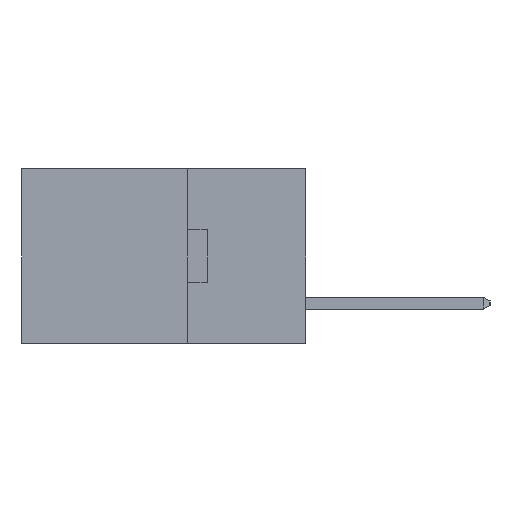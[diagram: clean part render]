
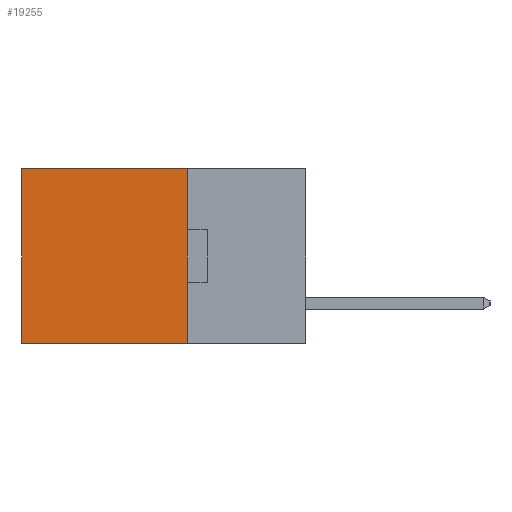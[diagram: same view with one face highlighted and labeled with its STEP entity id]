
A CAD part, left-side view. The second image highlights one B-rep face of the part: STEP entity #19255.
In plain terms, the highlighted planar face has unit normal (-1, 0, 0).
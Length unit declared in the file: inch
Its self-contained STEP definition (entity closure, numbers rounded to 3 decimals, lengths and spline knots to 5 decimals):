
#3061 = VERTEX_POINT ( 'NONE', #18362 ) ;
#4437 = FACE_OUTER_BOUND ( 'NONE', #25617, .T. ) ;
#4675 = CARTESIAN_POINT ( 'NONE',  ( 0.2615, 0.25, -0.37 ) ) ;
#6828 = VERTEX_POINT ( 'NONE', #25820 ) ;
#7215 = EDGE_CURVE ( 'NONE', #6828, #13916, #17630, .T. ) ;
#7653 = EDGE_CURVE ( 'NONE', #15940, #13916, #16345, .T. ) ;
#8813 = PLANE ( 'NONE',  #10673 ) ;
#8828 = ORIENTED_EDGE ( 'NONE', *, *, #11333, .F. ) ;
#10325 = VECTOR ( 'NONE', #12935, 39.37008 ) ;
#10673 = AXIS2_PLACEMENT_3D ( 'NONE', #23127, #10927, #25116 ) ;
#10927 = DIRECTION ( 'NONE',  ( 1., 0., 0. ) ) ;
#11333 = EDGE_CURVE ( 'NONE', #3061, #15940, #19306, .T. ) ;
#11552 = VECTOR ( 'NONE', #21786, 39.37008 ) ;
#12205 = LINE ( 'NONE', #13214, #17010 ) ;
#12935 = DIRECTION ( 'NONE',  ( 0., 0., -1. ) ) ;
#13214 = CARTESIAN_POINT ( 'NONE',  ( 0.2615, 0.25, 0. ) ) ;
#13916 = VERTEX_POINT ( 'NONE', #17057 ) ;
#15294 = DIRECTION ( 'NONE',  ( 0., 1., 0. ) ) ;
#15366 = ORIENTED_EDGE ( 'NONE', *, *, #24944, .T. ) ;
#15718 = VECTOR ( 'NONE', #16014, 39.37008 ) ;
#15844 = CARTESIAN_POINT ( 'NONE',  ( 0.2615, 0.25, -0.37 ) ) ;
#15940 = VERTEX_POINT ( 'NONE', #16402 ) ;
#16014 = DIRECTION ( 'NONE',  ( 0., 1., 0. ) ) ;
#16345 = LINE ( 'NONE', #15844, #15718 ) ;
#16402 = CARTESIAN_POINT ( 'NONE',  ( 0.2615, 0.25, -0.37 ) ) ;
#17010 = VECTOR ( 'NONE', #15294, 39.37008 ) ;
#17057 = CARTESIAN_POINT ( 'NONE',  ( 0.2615, 0.6, -0.37 ) ) ;
#17630 = LINE ( 'NONE', #21534, #11552 ) ;
#18362 = CARTESIAN_POINT ( 'NONE',  ( 0.2615, 0.25, 0. ) ) ;
#19255 = ADVANCED_FACE ( 'NONE', ( #4437 ), #8813, .F. ) ;
#19306 = LINE ( 'NONE', #4675, #10325 ) ;
#19738 = ORIENTED_EDGE ( 'NONE', *, *, #7215, .T. ) ;
#21534 = CARTESIAN_POINT ( 'NONE',  ( 0.2615, 0.6, -0.37 ) ) ;
#21786 = DIRECTION ( 'NONE',  ( 0., 0., -1. ) ) ;
#22882 = ORIENTED_EDGE ( 'NONE', *, *, #7653, .F. ) ;
#23127 = CARTESIAN_POINT ( 'NONE',  ( 0.2615, 0.25, -0.37 ) ) ;
#24944 = EDGE_CURVE ( 'NONE', #3061, #6828, #12205, .T. ) ;
#25116 = DIRECTION ( 'NONE',  ( 0., 0., -1. ) ) ;
#25617 = EDGE_LOOP ( 'NONE', ( #19738, #22882, #8828, #15366 ) ) ;
#25820 = CARTESIAN_POINT ( 'NONE',  ( 0.2615, 0.6, 0. ) ) ;
